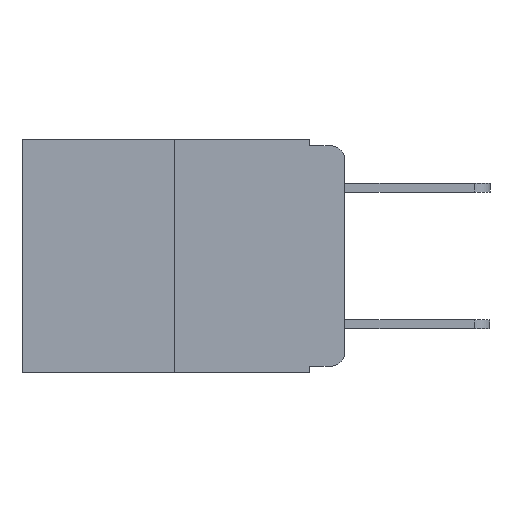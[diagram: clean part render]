
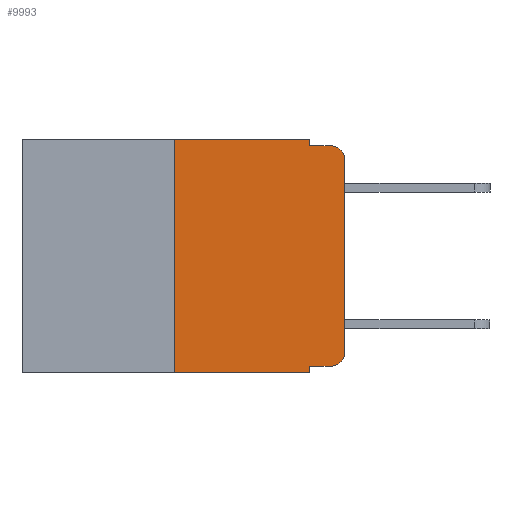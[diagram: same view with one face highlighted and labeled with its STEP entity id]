
A CAD part, left-side view. The second image highlights one B-rep face of the part: STEP entity #9993.
In plain terms, the highlighted planar face has unit normal (-1, 0, 0).
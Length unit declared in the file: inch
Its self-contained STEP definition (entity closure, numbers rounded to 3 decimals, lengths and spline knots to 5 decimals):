
#10 = EDGE_CURVE ( 'NONE', #780, #1953, #8728, .T. ) ;
#103 = DIRECTION ( 'NONE',  ( -1., 0., 0. ) ) ;
#247 = DIRECTION ( 'NONE',  ( 0., 0., 1. ) ) ;
#254 = VECTOR ( 'NONE', #4103, 39.37008 ) ;
#272 = DIRECTION ( 'NONE',  ( 0., 0., -1. ) ) ;
#408 = PLANE ( 'NONE',  #7207 ) ;
#425 = CARTESIAN_POINT ( 'NONE',  ( 0., 0.051, -0.333 ) ) ;
#653 = EDGE_CURVE ( 'NONE', #1571, #10168, #2914, .T. ) ;
#744 = CARTESIAN_POINT ( 'NONE',  ( 0., 0.25, 0. ) ) ;
#780 = VERTEX_POINT ( 'NONE', #4325 ) ;
#901 = LINE ( 'NONE', #2420, #9041 ) ;
#954 = CARTESIAN_POINT ( 'NONE',  ( 0., 0.051, 0. ) ) ;
#996 = CARTESIAN_POINT ( 'NONE',  ( 0., 0.051, -0.333 ) ) ;
#1052 = CARTESIAN_POINT ( 'NONE',  ( 0., 0., -0.313 ) ) ;
#1094 = ORIENTED_EDGE ( 'NONE', *, *, #6458, .F. ) ;
#1220 = EDGE_CURVE ( 'NONE', #7957, #1468, #2369, .T. ) ;
#1225 = CARTESIAN_POINT ( 'NONE',  ( 0., 0.02, -0.03 ) ) ;
#1303 = CARTESIAN_POINT ( 'NONE',  ( 0., 0., -0.03 ) ) ;
#1309 = VERTEX_POINT ( 'NONE', #425 ) ;
#1468 = VERTEX_POINT ( 'NONE', #7684 ) ;
#1571 = VERTEX_POINT ( 'NONE', #8740 ) ;
#1953 = VERTEX_POINT ( 'NONE', #1052 ) ;
#2183 = VERTEX_POINT ( 'NONE', #10005 ) ;
#2369 = LINE ( 'NONE', #744, #6702 ) ;
#2420 = CARTESIAN_POINT ( 'NONE',  ( 0., 0.051, -0.01 ) ) ;
#2442 = AXIS2_PLACEMENT_3D ( 'NONE', #1225, #103, #272 ) ;
#2509 = EDGE_CURVE ( 'NONE', #7957, #5140, #7504, .T. ) ;
#2841 = AXIS2_PLACEMENT_3D ( 'NONE', #8845, #7935, #7891 ) ;
#2905 = FACE_OUTER_BOUND ( 'NONE', #6569, .T. ) ;
#2914 = LINE ( 'NONE', #954, #9024 ) ;
#3010 = DIRECTION ( 'NONE',  ( 1., 0., 0. ) ) ;
#3079 = LINE ( 'NONE', #7918, #7471 ) ;
#3085 = VECTOR ( 'NONE', #3240, 39.37008 ) ;
#3240 = DIRECTION ( 'NONE',  ( 0., 0., 1. ) ) ;
#3250 = ORIENTED_EDGE ( 'NONE', *, *, #5857, .T. ) ;
#3373 = ORIENTED_EDGE ( 'NONE', *, *, #653, .F. ) ;
#3926 = ORIENTED_EDGE ( 'NONE', *, *, #1220, .F. ) ;
#4103 = DIRECTION ( 'NONE',  ( 0., -1., 0. ) ) ;
#4325 = CARTESIAN_POINT ( 'NONE',  ( 0., 0.02, -0.333 ) ) ;
#4466 = ORIENTED_EDGE ( 'NONE', *, *, #10, .T. ) ;
#4545 = CARTESIAN_POINT ( 'NONE',  ( 0., 0., 0. ) ) ;
#4555 = CIRCLE ( 'NONE', #2442, 0.02 ) ;
#4606 = CARTESIAN_POINT ( 'NONE',  ( 0., 0.473, 0. ) ) ;
#4709 = ORIENTED_EDGE ( 'NONE', *, *, #5318, .F. ) ;
#4859 = EDGE_CURVE ( 'NONE', #1953, #8936, #5308, .T. ) ;
#4879 = CARTESIAN_POINT ( 'NONE',  ( 0., 0.051, -0.01 ) ) ;
#4922 = EDGE_CURVE ( 'NONE', #1468, #1571, #8756, .T. ) ;
#5140 = VERTEX_POINT ( 'NONE', #6936 ) ;
#5196 = DIRECTION ( 'NONE',  ( 0., 0., -1. ) ) ;
#5273 = DIRECTION ( 'NONE',  ( 0., -1., 0. ) ) ;
#5308 = LINE ( 'NONE', #4545, #3085 ) ;
#5318 = EDGE_CURVE ( 'NONE', #1309, #5140, #3079, .T. ) ;
#5400 = EDGE_CURVE ( 'NONE', #8936, #2183, #4555, .T. ) ;
#5611 = DIRECTION ( 'NONE',  ( 0., -1., 0. ) ) ;
#5651 = CARTESIAN_POINT ( 'NONE',  ( 0., 0.473, -0.343 ) ) ;
#5857 = EDGE_CURVE ( 'NONE', #1309, #780, #8950, .T. ) ;
#6184 = ORIENTED_EDGE ( 'NONE', *, *, #4859, .T. ) ;
#6458 = EDGE_CURVE ( 'NONE', #10168, #2183, #901, .T. ) ;
#6569 = EDGE_LOOP ( 'NONE', ( #6184, #7292, #1094, #3373, #9669, #3926, #9888, #4709, #3250, #4466 ) ) ;
#6702 = VECTOR ( 'NONE', #247, 39.37008 ) ;
#6936 = CARTESIAN_POINT ( 'NONE',  ( 0., 0.051, -0.343 ) ) ;
#7056 = VECTOR ( 'NONE', #8812, 39.37008 ) ;
#7075 = CARTESIAN_POINT ( 'NONE',  ( 0., 0.25, -0.343 ) ) ;
#7207 = AXIS2_PLACEMENT_3D ( 'NONE', #7667, #3010, #8423 ) ;
#7292 = ORIENTED_EDGE ( 'NONE', *, *, #5400, .T. ) ;
#7293 = VECTOR ( 'NONE', #5611, 39.37008 ) ;
#7471 = VECTOR ( 'NONE', #9481, 39.37008 ) ;
#7504 = LINE ( 'NONE', #5651, #7293 ) ;
#7667 = CARTESIAN_POINT ( 'NONE',  ( 0., 0.473, 0. ) ) ;
#7684 = CARTESIAN_POINT ( 'NONE',  ( 0., 0.25, 0. ) ) ;
#7891 = DIRECTION ( 'NONE',  ( 0., 0., -1. ) ) ;
#7918 = CARTESIAN_POINT ( 'NONE',  ( 0., 0.051, 0. ) ) ;
#7935 = DIRECTION ( 'NONE',  ( -1., 0., 0. ) ) ;
#7957 = VERTEX_POINT ( 'NONE', #7075 ) ;
#8423 = DIRECTION ( 'NONE',  ( 0., 0., -1. ) ) ;
#8728 = CIRCLE ( 'NONE', #2841, 0.02 ) ;
#8740 = CARTESIAN_POINT ( 'NONE',  ( 0., 0.051, 0. ) ) ;
#8756 = LINE ( 'NONE', #4606, #254 ) ;
#8812 = DIRECTION ( 'NONE',  ( 0., -1., 0. ) ) ;
#8845 = CARTESIAN_POINT ( 'NONE',  ( 0., 0.02, -0.313 ) ) ;
#8936 = VERTEX_POINT ( 'NONE', #1303 ) ;
#8950 = LINE ( 'NONE', #996, #7056 ) ;
#9024 = VECTOR ( 'NONE', #5196, 39.37008 ) ;
#9041 = VECTOR ( 'NONE', #5273, 39.37008 ) ;
#9481 = DIRECTION ( 'NONE',  ( 0., 0., -1. ) ) ;
#9669 = ORIENTED_EDGE ( 'NONE', *, *, #4922, .F. ) ;
#9888 = ORIENTED_EDGE ( 'NONE', *, *, #2509, .T. ) ;
#9993 = ADVANCED_FACE ( 'NONE', ( #2905 ), #408, .F. ) ;
#10005 = CARTESIAN_POINT ( 'NONE',  ( 0., 0.02, -0.01 ) ) ;
#10168 = VERTEX_POINT ( 'NONE', #4879 ) ;
